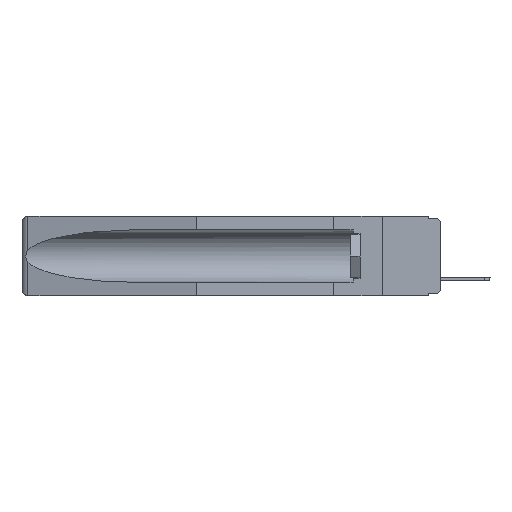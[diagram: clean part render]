
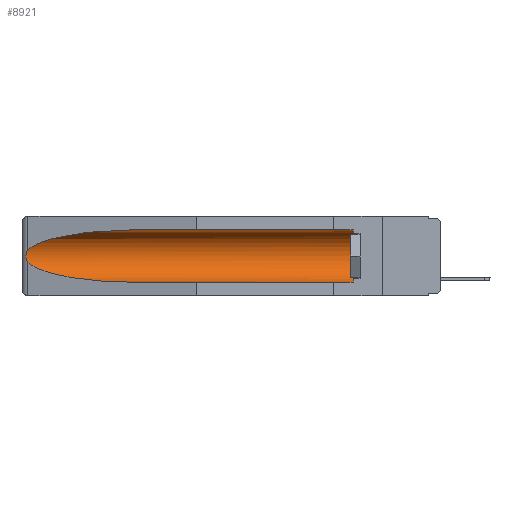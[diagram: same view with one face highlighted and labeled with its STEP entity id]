
A CAD part, left-side view. The second image highlights one B-rep face of the part: STEP entity #8921.
In plain terms, the highlighted cylindrical face has radius 2.857 mm (diameter 5.715 mm), a partial arc.
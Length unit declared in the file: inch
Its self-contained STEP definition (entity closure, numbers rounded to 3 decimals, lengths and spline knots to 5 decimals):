
#479 = LINE ( 'NONE', #16324, #20430 ) ;
#500 = EDGE_CURVE ( 'NONE', #12830, #21788, #2109, .T. ) ;
#556 = CARTESIAN_POINT ( 'NONE',  ( 0.155, 1.07973, -0.059 ) ) ;
#734 = EDGE_CURVE ( 'NONE', #7009, #5869, #5414, .T. ) ;
#1206 = VECTOR ( 'NONE', #3288, 39.37008 ) ;
#2067 = CARTESIAN_POINT ( 'NONE',  ( 0.21114, 1.30732, -0.284 ) ) ;
#2109 = CIRCLE ( 'NONE', #12135, 0.1125 ) ;
#3288 = DIRECTION ( 'NONE',  ( 0., 1., 0. ) ) ;
#3314 = CARTESIAN_POINT ( 'NONE',  ( 0.26597, 1.5296, -0.19026 ) ) ;
#3869 = EDGE_CURVE ( 'NONE', #21788, #21937, #8762, .T. ) ;
#5274 = CARTESIAN_POINT ( 'NONE',  ( 0.26654, 1.53092, -0.15636 ) ) ;
#5398 = CARTESIAN_POINT ( 'NONE',  ( 0.2673, 1.53269, -0.17917 ) ) ;
#5414 =( BOUNDED_CURVE ( )  B_SPLINE_CURVE ( 3, ( #17764, #12542, #2067, #8924 ),
 .UNSPECIFIED., .F., .T. ) 
 B_SPLINE_CURVE_WITH_KNOTS ( ( 4, 4 ),
 ( 0.1948, 1.5708 ),
 .UNSPECIFIED. ) 
 CURVE ( )  GEOMETRIC_REPRESENTATION_ITEM ( )  RATIONAL_B_SPLINE_CURVE ( ( 1., 0.848, 0.848, 1. ) ) 
 REPRESENTATION_ITEM ( '' )  );
#5683 = B_SPLINE_CURVE_WITH_KNOTS ( 'NONE', 3,
 ( #8434, #19147, #5274, #15661, #13798, #15788, #5398, #20889, #3314, #17624 ),
 .UNSPECIFIED., .F., .F.,
 ( 4, 2, 2, 2, 4 ),
 ( 0., 0.00029, 0.00058, 0.00087, 0.00117 ),
 .UNSPECIFIED. ) ;
#5869 = VERTEX_POINT ( 'NONE', #22770 ) ;
#5900 = CARTESIAN_POINT ( 'NONE',  ( 0.26537, 1.52718, -0.14972 ) ) ;
#6291 = CARTESIAN_POINT ( 'NONE',  ( 0.155, 1.07973, -0.059 ) ) ;
#6788 = FACE_OUTER_BOUND ( 'NONE', #16803, .T. ) ;
#7009 = VERTEX_POINT ( 'NONE', #9993 ) ;
#7596 = DIRECTION ( 'NONE',  ( 0., 1., 0. ) ) ;
#7672 = CARTESIAN_POINT ( 'NONE',  ( 0.21114, 1.30732, -0.059 ) ) ;
#8019 = CARTESIAN_POINT ( 'NONE',  ( 0.155, 0.126, -0.1715 ) ) ;
#8434 = CARTESIAN_POINT ( 'NONE',  ( 0.26537, 1.52718, -0.14972 ) ) ;
#8640 = CARTESIAN_POINT ( 'NONE',  ( 0.155, -0.30754, -0.1715 ) ) ;
#8723 = ORIENTED_EDGE ( 'NONE', *, *, #14786, .F. ) ;
#8762 = LINE ( 'NONE', #12808, #1206 ) ;
#8921 = ADVANCED_FACE ( 'NONE', ( #6788 ), #10395, .F. ) ;
#8924 = CARTESIAN_POINT ( 'NONE',  ( 0.155, 1.07973, -0.284 ) ) ;
#9125 = CARTESIAN_POINT ( 'NONE',  ( 0.155, 0.126, -0.284 ) ) ;
#9832 = AXIS2_PLACEMENT_3D ( 'NONE', #8640, #17712, #13896 ) ;
#9993 = CARTESIAN_POINT ( 'NONE',  ( 0.26537, 1.52718, -0.19328 ) ) ;
#10395 = CYLINDRICAL_SURFACE ( 'NONE', #9832, 0.1125 ) ;
#10773 = ORIENTED_EDGE ( 'NONE', *, *, #734, .T. ) ;
#11255 = EDGE_CURVE ( 'NONE', #21937, #13546, #15695, .T. ) ;
#11406 = ORIENTED_EDGE ( 'NONE', *, *, #11255, .T. ) ;
#12135 = AXIS2_PLACEMENT_3D ( 'NONE', #8019, #15131, #18704 ) ;
#12542 = CARTESIAN_POINT ( 'NONE',  ( 0.25451, 1.48313, -0.24835 ) ) ;
#12808 = CARTESIAN_POINT ( 'NONE',  ( 0.155, -0.30754, -0.059 ) ) ;
#12830 = VERTEX_POINT ( 'NONE', #9125 ) ;
#13546 = VERTEX_POINT ( 'NONE', #19044 ) ;
#13798 = CARTESIAN_POINT ( 'NONE',  ( 0.2675, 1.53308, -0.16763 ) ) ;
#13896 = DIRECTION ( 'NONE',  ( 0., 0., 1. ) ) ;
#14786 = EDGE_CURVE ( 'NONE', #12830, #5869, #479, .T. ) ;
#14887 = CARTESIAN_POINT ( 'NONE',  ( 0.25451, 1.48313, -0.09465 ) ) ;
#14954 = ORIENTED_EDGE ( 'NONE', *, *, #500, .T. ) ;
#15131 = DIRECTION ( 'NONE',  ( 0., -1., 0. ) ) ;
#15661 = CARTESIAN_POINT ( 'NONE',  ( 0.2673, 1.5327, -0.16383 ) ) ;
#15695 =( BOUNDED_CURVE ( )  B_SPLINE_CURVE ( 3, ( #556, #7672, #14887, #5900 ),
 .UNSPECIFIED., .F., .T. ) 
 B_SPLINE_CURVE_WITH_KNOTS ( ( 4, 4 ),
 ( 4.71239, 6.08839 ),
 .UNSPECIFIED. ) 
 CURVE ( )  GEOMETRIC_REPRESENTATION_ITEM ( )  RATIONAL_B_SPLINE_CURVE ( ( 1., 0.848, 0.848, 1. ) ) 
 REPRESENTATION_ITEM ( '' )  );
#15788 = CARTESIAN_POINT ( 'NONE',  ( 0.2675, 1.53308, -0.17534 ) ) ;
#16100 = CARTESIAN_POINT ( 'NONE',  ( 0.155, 0.126, -0.059 ) ) ;
#16116 = ORIENTED_EDGE ( 'NONE', *, *, #3869, .T. ) ;
#16324 = CARTESIAN_POINT ( 'NONE',  ( 0.155, -0.30754, -0.284 ) ) ;
#16803 = EDGE_LOOP ( 'NONE', ( #11406, #19292, #10773, #8723, #14954, #16116 ) ) ;
#17624 = CARTESIAN_POINT ( 'NONE',  ( 0.26537, 1.52718, -0.19328 ) ) ;
#17712 = DIRECTION ( 'NONE',  ( 0., 1., 0. ) ) ;
#17764 = CARTESIAN_POINT ( 'NONE',  ( 0.26537, 1.52718, -0.19328 ) ) ;
#18704 = DIRECTION ( 'NONE',  ( 0., 0., 1. ) ) ;
#19044 = CARTESIAN_POINT ( 'NONE',  ( 0.26537, 1.52718, -0.14972 ) ) ;
#19147 = CARTESIAN_POINT ( 'NONE',  ( 0.26597, 1.52961, -0.15275 ) ) ;
#19292 = ORIENTED_EDGE ( 'NONE', *, *, #19895, .T. ) ;
#19895 = EDGE_CURVE ( 'NONE', #13546, #7009, #5683, .T. ) ;
#20430 = VECTOR ( 'NONE', #7596, 39.37008 ) ;
#20889 = CARTESIAN_POINT ( 'NONE',  ( 0.26655, 1.53094, -0.18657 ) ) ;
#21788 = VERTEX_POINT ( 'NONE', #16100 ) ;
#21937 = VERTEX_POINT ( 'NONE', #6291 ) ;
#22770 = CARTESIAN_POINT ( 'NONE',  ( 0.155, 1.07973, -0.284 ) ) ;
